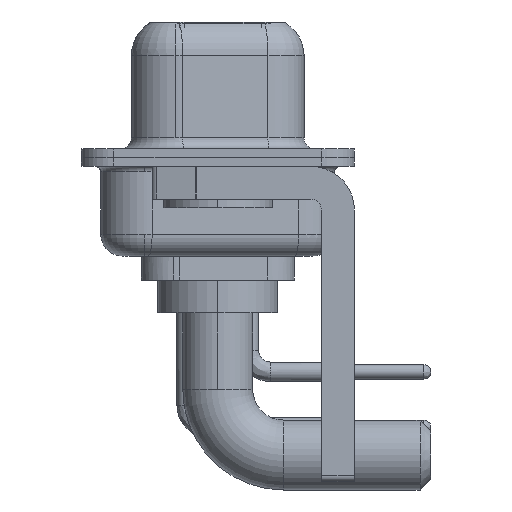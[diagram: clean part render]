
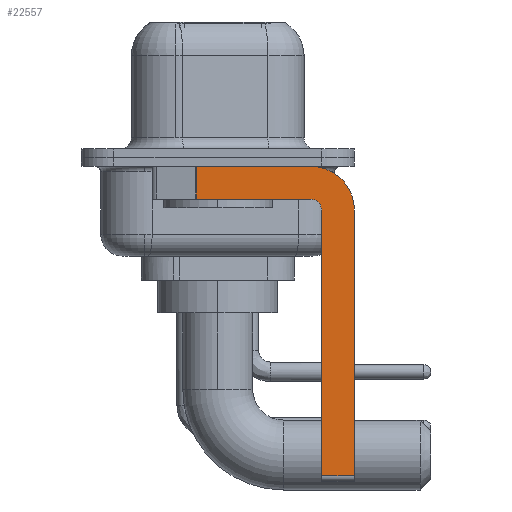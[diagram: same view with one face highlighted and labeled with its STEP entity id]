
A CAD part, left-side view. The second image highlights one B-rep face of the part: STEP entity #22557.
In plain terms, the highlighted planar face has unit normal (-1, 0, 0).
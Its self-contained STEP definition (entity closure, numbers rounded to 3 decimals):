
#7 = CARTESIAN_POINT ( 'NONE',  ( -2.9, -4.25, -0.4 ) ) ;
#90 = ORIENTED_EDGE ( 'NONE', *, *, #16722, .T. ) ;
#184 = EDGE_CURVE ( 'NONE', #2756, #6857, #17353, .T. ) ;
#1155 = DIRECTION ( 'NONE',  ( -1., 0., 0. ) ) ;
#1384 = VECTOR ( 'NONE', #18850, 1000. ) ;
#2220 = LINE ( 'NONE', #4174, #4937 ) ;
#2505 = VERTEX_POINT ( 'NONE', #2657 ) ;
#2615 = VECTOR ( 'NONE', #16666, 1000. ) ;
#2657 = CARTESIAN_POINT ( 'NONE',  ( -2.9, -4.75, -14.55 ) ) ;
#2756 = VERTEX_POINT ( 'NONE', #6929 ) ;
#3011 = VERTEX_POINT ( 'NONE', #12198 ) ;
#3367 = EDGE_CURVE ( 'NONE', #3011, #17427, #8111, .T. ) ;
#4174 = CARTESIAN_POINT ( 'NONE',  ( -2.9, -4.25, -14.55 ) ) ;
#4289 = ORIENTED_EDGE ( 'NONE', *, *, #12205, .F. ) ;
#4937 = VECTOR ( 'NONE', #12638, 1000. ) ;
#5264 = CARTESIAN_POINT ( 'NONE',  ( -2.9, -4.25, -2.4 ) ) ;
#5642 = EDGE_LOOP ( 'NONE', ( #6330, #90, #14728, #21946, #16285, #22155, #4289, #22040 ) ) ;
#6330 = ORIENTED_EDGE ( 'NONE', *, *, #3367, .F. ) ;
#6634 = DIRECTION ( 'NONE',  ( 0., 0., -1. ) ) ;
#6857 = VERTEX_POINT ( 'NONE', #10993 ) ;
#6929 = CARTESIAN_POINT ( 'NONE',  ( -2.9, -4.25, -1.9 ) ) ;
#7002 = DIRECTION ( 'NONE',  ( 1., 0., 0. ) ) ;
#8091 = DIRECTION ( 'NONE',  ( 0., 0., 1. ) ) ;
#8111 = LINE ( 'NONE', #15168, #2615 ) ;
#8887 = VECTOR ( 'NONE', #6634, 1000. ) ;
#9424 = CARTESIAN_POINT ( 'NONE',  ( -2.9, -6.25, -2.4 ) ) ;
#9907 = VECTOR ( 'NONE', #14418, 1000. ) ;
#10224 = CARTESIAN_POINT ( 'NONE',  ( -2.9, 0.978, -1.9 ) ) ;
#10725 = EDGE_CURVE ( 'NONE', #17427, #16650, #16861, .T. ) ;
#10993 = CARTESIAN_POINT ( 'NONE',  ( -2.9, 0.978, -1.9 ) ) ;
#11131 = EDGE_CURVE ( 'NONE', #2505, #14614, #22396, .T. ) ;
#11198 = LINE ( 'NONE', #12939, #9907 ) ;
#11307 = CIRCLE ( 'NONE', #13858, 0.5 ) ;
#11691 = DIRECTION ( 'NONE',  ( 0., 0., -1. ) ) ;
#11833 = DIRECTION ( 'NONE',  ( 0., 0., 1. ) ) ;
#12198 = CARTESIAN_POINT ( 'NONE',  ( -2.9, 0.978, -0.4 ) ) ;
#12205 = EDGE_CURVE ( 'NONE', #16650, #16390, #11198, .T. ) ;
#12638 = DIRECTION ( 'NONE',  ( 0., -1., 0. ) ) ;
#12939 = CARTESIAN_POINT ( 'NONE',  ( -2.9, -6.25, -2.4 ) ) ;
#13098 = CARTESIAN_POINT ( 'NONE',  ( -2.9, -4.25, -2.4 ) ) ;
#13135 = AXIS2_PLACEMENT_3D ( 'NONE', #13098, #20095, #11691 ) ;
#13858 = AXIS2_PLACEMENT_3D ( 'NONE', #20205, #1155, #8091 ) ;
#14418 = DIRECTION ( 'NONE',  ( 0., 0., -1. ) ) ;
#14614 = VERTEX_POINT ( 'NONE', #15164 ) ;
#14662 = AXIS2_PLACEMENT_3D ( 'NONE', #5264, #7002, #21179 ) ;
#14728 = ORIENTED_EDGE ( 'NONE', *, *, #184, .F. ) ;
#15164 = CARTESIAN_POINT ( 'NONE',  ( -2.9, -4.75, -2.4 ) ) ;
#15168 = CARTESIAN_POINT ( 'NONE',  ( -2.9, 3., -0.4 ) ) ;
#15262 = FACE_OUTER_BOUND ( 'NONE', #5642, .T. ) ;
#15297 = CARTESIAN_POINT ( 'NONE',  ( -2.9, -4.25, -1.9 ) ) ;
#16285 = ORIENTED_EDGE ( 'NONE', *, *, #11131, .F. ) ;
#16390 = VERTEX_POINT ( 'NONE', #16939 ) ;
#16650 = VERTEX_POINT ( 'NONE', #9424 ) ;
#16666 = DIRECTION ( 'NONE',  ( 0., -1., 0. ) ) ;
#16722 = EDGE_CURVE ( 'NONE', #3011, #6857, #22186, .T. ) ;
#16861 = CIRCLE ( 'NONE', #14662, 2. ) ;
#16939 = CARTESIAN_POINT ( 'NONE',  ( -2.9, -6.25, -14.55 ) ) ;
#17353 = LINE ( 'NONE', #15297, #1384 ) ;
#17427 = VERTEX_POINT ( 'NONE', #7 ) ;
#18850 = DIRECTION ( 'NONE',  ( 0., 1., 0. ) ) ;
#19075 = VECTOR ( 'NONE', #11833, 1000. ) ;
#20095 = DIRECTION ( 'NONE',  ( 1., 0., 0. ) ) ;
#20205 = CARTESIAN_POINT ( 'NONE',  ( -2.9, -4.25, -2.4 ) ) ;
#21069 = EDGE_CURVE ( 'NONE', #2505, #16390, #2220, .T. ) ;
#21179 = DIRECTION ( 'NONE',  ( 0., 0., -1. ) ) ;
#21946 = ORIENTED_EDGE ( 'NONE', *, *, #22553, .F. ) ;
#22040 = ORIENTED_EDGE ( 'NONE', *, *, #10725, .F. ) ;
#22155 = ORIENTED_EDGE ( 'NONE', *, *, #21069, .T. ) ;
#22186 = LINE ( 'NONE', #10224, #8887 ) ;
#22244 = PLANE ( 'NONE',  #13135 ) ;
#22282 = CARTESIAN_POINT ( 'NONE',  ( -2.9, -4.75, -14.8 ) ) ;
#22396 = LINE ( 'NONE', #22282, #19075 ) ;
#22553 = EDGE_CURVE ( 'NONE', #14614, #2756, #11307, .T. ) ;
#22557 = ADVANCED_FACE ( 'NONE', ( #15262 ), #22244, .F. ) ;
